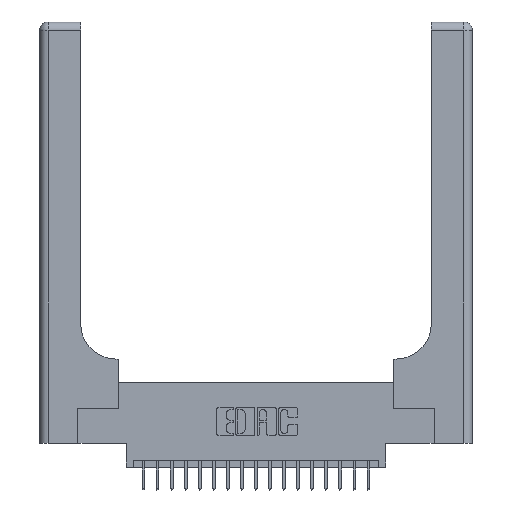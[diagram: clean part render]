
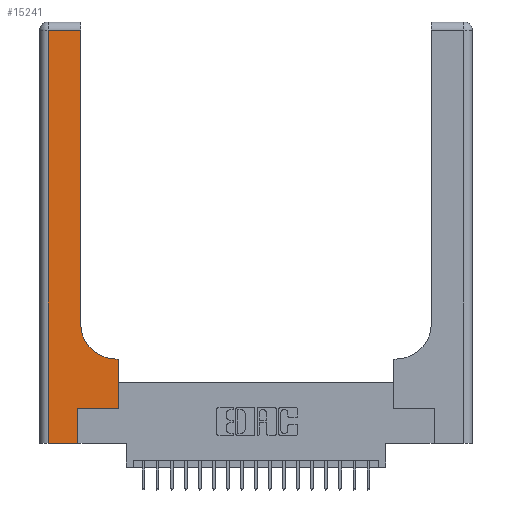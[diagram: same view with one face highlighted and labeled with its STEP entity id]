
A CAD part, top view. The second image highlights one B-rep face of the part: STEP entity #15241.
In plain terms, the highlighted planar face has unit normal (0, 0, 1).
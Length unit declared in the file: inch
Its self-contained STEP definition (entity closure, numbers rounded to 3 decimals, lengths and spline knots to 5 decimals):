
#1032 = LINE ( 'NONE', #8482, #14766 ) ;
#1230 = ORIENTED_EDGE ( 'NONE', *, *, #21813, .T. ) ;
#1712 = CARTESIAN_POINT ( 'NONE',  ( 0., 0., 0.37 ) ) ;
#2172 = LINE ( 'NONE', #18351, #6817 ) ;
#2193 = VERTEX_POINT ( 'NONE', #19960 ) ;
#2403 = CARTESIAN_POINT ( 'NONE',  ( 0.5415, 0.85, 0.37 ) ) ;
#2624 = DIRECTION ( 'NONE',  ( 0., 0., -1. ) ) ;
#2809 = EDGE_CURVE ( 'NONE', #16494, #18419, #12163, .T. ) ;
#2850 = ORIENTED_EDGE ( 'NONE', *, *, #16536, .T. ) ;
#3286 = DIRECTION ( 'NONE',  ( -1., 0., 0. ) ) ;
#3446 = LINE ( 'NONE', #10871, #17061 ) ;
#3929 = LINE ( 'NONE', #9407, #9055 ) ;
#4202 = DIRECTION ( 'NONE',  ( 1., 0., 0. ) ) ;
#4546 = VECTOR ( 'NONE', #5195, 39.37008 ) ;
#4836 = FACE_OUTER_BOUND ( 'NONE', #7377, .T. ) ;
#4900 = CARTESIAN_POINT ( 'NONE',  ( 0.269, 0.25, 0.37 ) ) ;
#5124 = ORIENTED_EDGE ( 'NONE', *, *, #15533, .T. ) ;
#5190 = VECTOR ( 'NONE', #19860, 39.37008 ) ;
#5195 = DIRECTION ( 'NONE',  ( 1., 0., 0. ) ) ;
#5438 = DIRECTION ( 'NONE',  ( -1., 0., 0. ) ) ;
#5823 = CARTESIAN_POINT ( 'NONE',  ( 0.5585, 0.6, 0.37 ) ) ;
#6751 = VERTEX_POINT ( 'NONE', #11917 ) ;
#6817 = VECTOR ( 'NONE', #14980, 39.37008 ) ;
#7153 = ORIENTED_EDGE ( 'NONE', *, *, #8656, .T. ) ;
#7377 = EDGE_LOOP ( 'NONE', ( #2850, #7153, #15650, #5124, #14327, #14570, #1230, #10503, #12038 ) ) ;
#7748 = CARTESIAN_POINT ( 'NONE',  ( 0., 3., 0.37 ) ) ;
#8022 = CARTESIAN_POINT ( 'NONE',  ( 0.5585, 0.25, 0.37 ) ) ;
#8482 = CARTESIAN_POINT ( 'NONE',  ( 0.2915, 0.6, 0.37 ) ) ;
#8656 = EDGE_CURVE ( 'NONE', #19225, #21821, #14848, .T. ) ;
#9055 = VECTOR ( 'NONE', #21158, 39.37008 ) ;
#9090 = VERTEX_POINT ( 'NONE', #4900 ) ;
#9407 = CARTESIAN_POINT ( 'NONE',  ( 0.2915, 3., 0.37 ) ) ;
#10205 = VECTOR ( 'NONE', #18896, 39.37008 ) ;
#10503 = ORIENTED_EDGE ( 'NONE', *, *, #20179, .T. ) ;
#10871 = CARTESIAN_POINT ( 'NONE',  ( 0.269, 0., 0.37 ) ) ;
#10879 = CARTESIAN_POINT ( 'NONE',  ( 0.2915, 0.85, 0.37 ) ) ;
#11742 = CARTESIAN_POINT ( 'NONE',  ( 0.2915, 2.94, 0.37 ) ) ;
#11840 = AXIS2_PLACEMENT_3D ( 'NONE', #7748, #2624, #14639 ) ;
#11917 = CARTESIAN_POINT ( 'NONE',  ( 0.5585, 0.25, 0.37 ) ) ;
#12038 = ORIENTED_EDGE ( 'NONE', *, *, #2809, .T. ) ;
#12163 = CIRCLE ( 'NONE', #15662, 0.25 ) ;
#13057 = LINE ( 'NONE', #1712, #4546 ) ;
#14327 = ORIENTED_EDGE ( 'NONE', *, *, #15092, .T. ) ;
#14419 = DIRECTION ( 'NONE',  ( 0., 0., -1. ) ) ;
#14570 = ORIENTED_EDGE ( 'NONE', *, *, #18009, .T. ) ;
#14639 = DIRECTION ( 'NONE',  ( -1., 0., 0. ) ) ;
#14766 = VECTOR ( 'NONE', #3286, 39.37008 ) ;
#14848 = LINE ( 'NONE', #20573, #18780 ) ;
#14944 = EDGE_CURVE ( 'NONE', #21821, #2193, #19656, .T. ) ;
#14980 = DIRECTION ( 'NONE',  ( 1., 0., 0. ) ) ;
#15092 = EDGE_CURVE ( 'NONE', #17250, #9090, #3446, .T. ) ;
#15241 = ADVANCED_FACE ( 'NONE', ( #4836 ), #19604, .F. ) ;
#15533 = EDGE_CURVE ( 'NONE', #2193, #17250, #13057, .T. ) ;
#15650 = ORIENTED_EDGE ( 'NONE', *, *, #14944, .T. ) ;
#15662 = AXIS2_PLACEMENT_3D ( 'NONE', #2403, #14419, #4202 ) ;
#16494 = VERTEX_POINT ( 'NONE', #16984 ) ;
#16501 = CARTESIAN_POINT ( 'NONE',  ( 0.06, 2.94, 0.37 ) ) ;
#16536 = EDGE_CURVE ( 'NONE', #18419, #19225, #3929, .T. ) ;
#16984 = CARTESIAN_POINT ( 'NONE',  ( 0.5415, 0.6, 0.37 ) ) ;
#17061 = VECTOR ( 'NONE', #17579, 39.37008 ) ;
#17234 = CARTESIAN_POINT ( 'NONE',  ( 0.06, 3., 0.37 ) ) ;
#17250 = VERTEX_POINT ( 'NONE', #19669 ) ;
#17579 = DIRECTION ( 'NONE',  ( 0., 1., 0. ) ) ;
#17744 = VERTEX_POINT ( 'NONE', #5823 ) ;
#18009 = EDGE_CURVE ( 'NONE', #9090, #6751, #2172, .T. ) ;
#18351 = CARTESIAN_POINT ( 'NONE',  ( 0.269, 0.25, 0.37 ) ) ;
#18419 = VERTEX_POINT ( 'NONE', #10879 ) ;
#18694 = LINE ( 'NONE', #8022, #5190 ) ;
#18780 = VECTOR ( 'NONE', #5438, 39.37008 ) ;
#18896 = DIRECTION ( 'NONE',  ( 0., -1., 0. ) ) ;
#19225 = VERTEX_POINT ( 'NONE', #11742 ) ;
#19604 = PLANE ( 'NONE',  #11840 ) ;
#19656 = LINE ( 'NONE', #17234, #10205 ) ;
#19669 = CARTESIAN_POINT ( 'NONE',  ( 0.269, 0., 0.37 ) ) ;
#19860 = DIRECTION ( 'NONE',  ( 0., 1., 0. ) ) ;
#19960 = CARTESIAN_POINT ( 'NONE',  ( 0.06, 0., 0.37 ) ) ;
#20179 = EDGE_CURVE ( 'NONE', #17744, #16494, #1032, .T. ) ;
#20573 = CARTESIAN_POINT ( 'NONE',  ( 0., 2.94, 0.37 ) ) ;
#21158 = DIRECTION ( 'NONE',  ( 0., 1., 0. ) ) ;
#21813 = EDGE_CURVE ( 'NONE', #6751, #17744, #18694, .T. ) ;
#21821 = VERTEX_POINT ( 'NONE', #16501 ) ;
